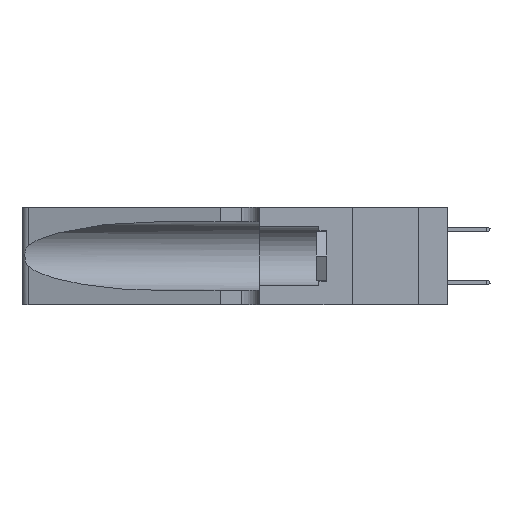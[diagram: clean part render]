
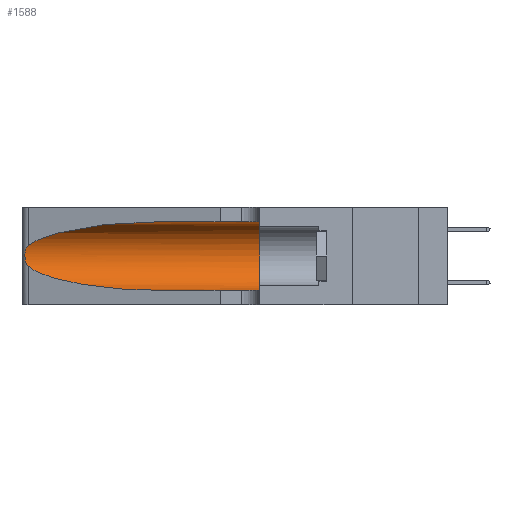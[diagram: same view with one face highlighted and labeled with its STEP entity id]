
A CAD part, left-side view. The second image highlights one B-rep face of the part: STEP entity #1588.
In plain terms, the highlighted cylindrical face has radius 3.308 mm (diameter 6.617 mm), a partial arc.
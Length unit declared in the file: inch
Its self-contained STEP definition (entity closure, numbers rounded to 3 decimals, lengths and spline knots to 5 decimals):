
#725 = CARTESIAN_POINT ( 'NONE',  ( 0.26075, 1.23896, 0.19203 ) ) ;
#1588 = ADVANCED_FACE ( 'NONE', ( #16753 ), #16148, .F. ) ;
#1713 = DIRECTION ( 'NONE',  ( 0., -1., 0. ) ) ;
#2266 = VECTOR ( 'NONE', #1713, 39.37008 ) ;
#2646 = VERTEX_POINT ( 'NONE', #11021 ) ;
#2727 = CARTESIAN_POINT ( 'NONE',  ( 0.25555, 1.22994, 0.2215 ) ) ;
#2822 = CARTESIAN_POINT ( 'NONE',  ( 0.26017, 1.23833, 0.17102 ) ) ;
#3042 = VERTEX_POINT ( 'NONE', #20235 ) ;
#3365 = AXIS2_PLACEMENT_3D ( 'NONE', #5950, #15876, #25482 ) ;
#3367 =( BOUNDED_CURVE ( )  B_SPLINE_CURVE ( 3, ( #9329, #11308, #24905, #13306 ),
 .UNSPECIFIED., .F., .T. ) 
 B_SPLINE_CURVE_WITH_KNOTS ( ( 4, 4 ),
 ( 1.5708, 2.84003 ),
 .UNSPECIFIED. ) 
 CURVE ( )  GEOMETRIC_REPRESENTATION_ITEM ( )  RATIONAL_B_SPLINE_CURVE ( ( 1., 0.87, 0.87, 1. ) ) 
 REPRESENTATION_ITEM ( '' )  );
#4081 = VERTEX_POINT ( 'NONE', #11621 ) ;
#4503 = EDGE_LOOP ( 'NONE', ( #9230, #15465, #20263, #4632, #21976, #4949 ) ) ;
#4561 = CARTESIAN_POINT ( 'NONE',  ( 0.1305, 0.35, 0.31525 ) ) ;
#4632 = ORIENTED_EDGE ( 'NONE', *, *, #6694, .T. ) ;
#4750 = CARTESIAN_POINT ( 'NONE',  ( 0.25487, 1.22718, 0.22369 ) ) ;
#4836 = CARTESIAN_POINT ( 'NONE',  ( 0.25789, 1.23486, 0.15765 ) ) ;
#4949 = ORIENTED_EDGE ( 'NONE', *, *, #23697, .F. ) ;
#5950 = CARTESIAN_POINT ( 'NONE',  ( 0.1305, 1.61858, 0.185 ) ) ;
#6694 = EDGE_CURVE ( 'NONE', #4081, #19573, #8257, .T. ) ;
#6817 = CARTESIAN_POINT ( 'NONE',  ( 0.1305, 1.61858, 0.31525 ) ) ;
#6897 = CARTESIAN_POINT ( 'NONE',  ( 0.25555, 1.22993, 0.14849 ) ) ;
#7514 = VERTEX_POINT ( 'NONE', #4561 ) ;
#7723 = CARTESIAN_POINT ( 'NONE',  ( 0.1305, 1.61858, 0.05475 ) ) ;
#8257 = LINE ( 'NONE', #7723, #2266 ) ;
#8290 = CARTESIAN_POINT ( 'NONE',  ( 0.1305, 0.72297, 0.31525 ) ) ;
#8398 = AXIS2_PLACEMENT_3D ( 'NONE', #9942, #23550, #11914 ) ;
#8812 = DIRECTION ( 'NONE',  ( 0., -1., 0. ) ) ;
#9230 = ORIENTED_EDGE ( 'NONE', *, *, #19632, .T. ) ;
#9329 = CARTESIAN_POINT ( 'NONE',  ( 0.1305, 0.72297, 0.31525 ) ) ;
#9942 = CARTESIAN_POINT ( 'NONE',  ( 0.1305, 0.35, 0.185 ) ) ;
#10781 = CARTESIAN_POINT ( 'NONE',  ( 0.25787, 1.23484, 0.2124 ) ) ;
#11021 = CARTESIAN_POINT ( 'NONE',  ( 0.25487, 1.22718, 0.22369 ) ) ;
#11133 = CARTESIAN_POINT ( 'NONE',  ( 0.1305, 0.35, 0.05475 ) ) ;
#11308 = CARTESIAN_POINT ( 'NONE',  ( 0.18966, 0.96281, 0.31525 ) ) ;
#11621 = CARTESIAN_POINT ( 'NONE',  ( 0.1305, 0.72297, 0.05475 ) ) ;
#11914 = DIRECTION ( 'NONE',  ( 0., 0., 1. ) ) ;
#12336 =( BOUNDED_CURVE ( )  B_SPLINE_CURVE ( 3, ( #22886, #20976, #24848, #13253 ),
 .UNSPECIFIED., .F., .T. ) 
 B_SPLINE_CURVE_WITH_KNOTS ( ( 4, 4 ),
 ( 3.44316, 4.71239 ),
 .UNSPECIFIED. ) 
 CURVE ( )  GEOMETRIC_REPRESENTATION_ITEM ( )  RATIONAL_B_SPLINE_CURVE ( ( 1., 0.87, 0.87, 1. ) ) 
 REPRESENTATION_ITEM ( '' )  );
#12777 = CARTESIAN_POINT ( 'NONE',  ( 0.26018, 1.23835, 0.19895 ) ) ;
#12813 = VECTOR ( 'NONE', #8812, 39.37008 ) ;
#12839 = EDGE_CURVE ( 'NONE', #7514, #19573, #13587, .T. ) ;
#13253 = CARTESIAN_POINT ( 'NONE',  ( 0.1305, 0.72297, 0.05475 ) ) ;
#13306 = CARTESIAN_POINT ( 'NONE',  ( 0.25487, 1.22718, 0.22369 ) ) ;
#13587 = CIRCLE ( 'NONE', #8398, 0.13025 ) ;
#14536 = B_SPLINE_CURVE_WITH_KNOTS ( 'NONE', 3,
 ( #4750, #2727, #22430, #10781, #24382, #12777, #725, #14755, #2822, #16679, #4836, #18653, #6897, #20595 ),
 .UNSPECIFIED., .F., .F.,
 ( 4, 2, 2, 2, 2, 2, 4 ),
 ( 0., 0.00027, 0.00053, 0.00107, 0.0016, 0.00187, 0.00214 ),
 .UNSPECIFIED. ) ;
#14755 = CARTESIAN_POINT ( 'NONE',  ( 0.26075, 1.23896, 0.178 ) ) ;
#15452 = EDGE_CURVE ( 'NONE', #2646, #3042, #14536, .T. ) ;
#15465 = ORIENTED_EDGE ( 'NONE', *, *, #15452, .T. ) ;
#15876 = DIRECTION ( 'NONE',  ( 0., -1., 0. ) ) ;
#16148 = CYLINDRICAL_SURFACE ( 'NONE', #3365, 0.13025 ) ;
#16679 = CARTESIAN_POINT ( 'NONE',  ( 0.25856, 1.23593, 0.16098 ) ) ;
#16753 = FACE_OUTER_BOUND ( 'NONE', #4503, .T. ) ;
#16994 = EDGE_CURVE ( 'NONE', #3042, #4081, #12336, .T. ) ;
#17837 = VERTEX_POINT ( 'NONE', #8290 ) ;
#18653 = CARTESIAN_POINT ( 'NONE',  ( 0.25639, 1.23186, 0.15144 ) ) ;
#19573 = VERTEX_POINT ( 'NONE', #11133 ) ;
#19632 = EDGE_CURVE ( 'NONE', #17837, #2646, #3367, .T. ) ;
#20235 = CARTESIAN_POINT ( 'NONE',  ( 0.25487, 1.22718, 0.14631 ) ) ;
#20263 = ORIENTED_EDGE ( 'NONE', *, *, #16994, .T. ) ;
#20595 = CARTESIAN_POINT ( 'NONE',  ( 0.25487, 1.22718, 0.14631 ) ) ;
#20976 = CARTESIAN_POINT ( 'NONE',  ( 0.2373, 1.15595, 0.08982 ) ) ;
#21976 = ORIENTED_EDGE ( 'NONE', *, *, #12839, .F. ) ;
#22430 = CARTESIAN_POINT ( 'NONE',  ( 0.25639, 1.23184, 0.21858 ) ) ;
#22886 = CARTESIAN_POINT ( 'NONE',  ( 0.25487, 1.22718, 0.14631 ) ) ;
#23100 = LINE ( 'NONE', #6817, #12813 ) ;
#23550 = DIRECTION ( 'NONE',  ( 0., 1., 0. ) ) ;
#23697 = EDGE_CURVE ( 'NONE', #17837, #7514, #23100, .T. ) ;
#24382 = CARTESIAN_POINT ( 'NONE',  ( 0.25854, 1.2359, 0.20912 ) ) ;
#24848 = CARTESIAN_POINT ( 'NONE',  ( 0.18966, 0.96281, 0.05475 ) ) ;
#24905 = CARTESIAN_POINT ( 'NONE',  ( 0.2373, 1.15595, 0.28018 ) ) ;
#25482 = DIRECTION ( 'NONE',  ( 0., 0., -1. ) ) ;
